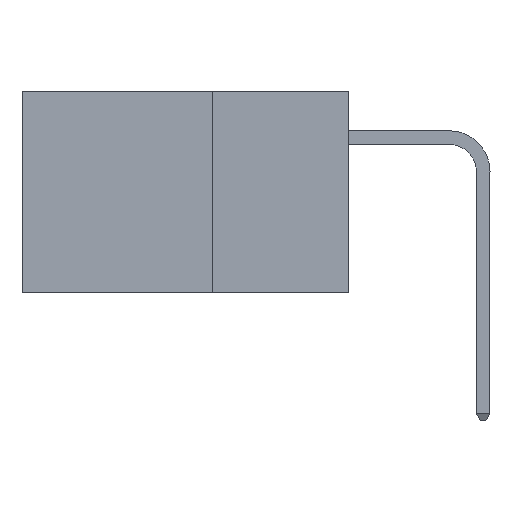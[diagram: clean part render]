
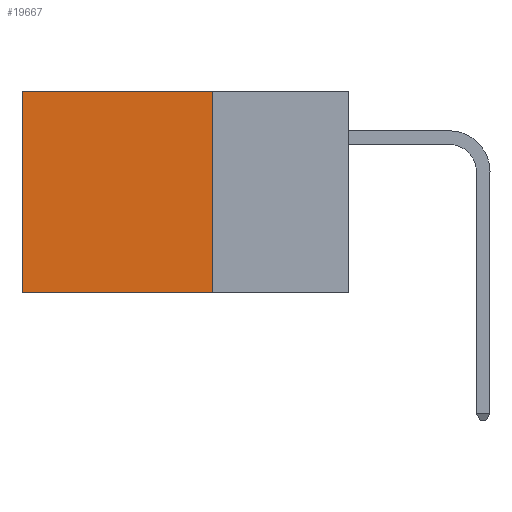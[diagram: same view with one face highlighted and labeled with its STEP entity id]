
A CAD part, left-side view. The second image highlights one B-rep face of the part: STEP entity #19667.
In plain terms, the highlighted planar face has unit normal (-1, 0, 0).
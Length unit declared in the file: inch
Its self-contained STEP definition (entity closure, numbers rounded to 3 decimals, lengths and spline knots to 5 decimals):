
#510 = VERTEX_POINT ( 'NONE', #16244 ) ;
#1344 = LINE ( 'NONE', #4701, #18742 ) ;
#1558 = CARTESIAN_POINT ( 'NONE',  ( 0.2875, 0.25, -0.37 ) ) ;
#2072 = CARTESIAN_POINT ( 'NONE',  ( 0.2875, 0.25, 0. ) ) ;
#2554 = ORIENTED_EDGE ( 'NONE', *, *, #17748, .T. ) ;
#4329 = LINE ( 'NONE', #9732, #13766 ) ;
#4585 = DIRECTION ( 'NONE',  ( 0., 1., 0. ) ) ;
#4683 = DIRECTION ( 'NONE',  ( 0., 0., -1. ) ) ;
#4701 = CARTESIAN_POINT ( 'NONE',  ( 0.2875, 0.25, -0.37 ) ) ;
#5340 = EDGE_CURVE ( 'NONE', #510, #19497, #20438, .T. ) ;
#6533 = CARTESIAN_POINT ( 'NONE',  ( 0.2875, 0.6, -0.37 ) ) ;
#7236 = DIRECTION ( 'NONE',  ( 0., 0., -1. ) ) ;
#8047 = DIRECTION ( 'NONE',  ( 0., 0., -1. ) ) ;
#8065 = FACE_OUTER_BOUND ( 'NONE', #16043, .T. ) ;
#8788 = VERTEX_POINT ( 'NONE', #9786 ) ;
#9732 = CARTESIAN_POINT ( 'NONE',  ( 0.2875, 0.6, 0. ) ) ;
#9786 = CARTESIAN_POINT ( 'NONE',  ( 0.2875, 0.6, 0. ) ) ;
#11157 = ORIENTED_EDGE ( 'NONE', *, *, #5340, .F. ) ;
#12168 = PLANE ( 'NONE',  #21202 ) ;
#13369 = ORIENTED_EDGE ( 'NONE', *, *, #16544, .T. ) ;
#13582 = VERTEX_POINT ( 'NONE', #6533 ) ;
#13766 = VECTOR ( 'NONE', #4683, 39.37008 ) ;
#14078 = VECTOR ( 'NONE', #4585, 39.37008 ) ;
#14238 = ORIENTED_EDGE ( 'NONE', *, *, #20639, .F. ) ;
#16010 = VECTOR ( 'NONE', #8047, 39.37008 ) ;
#16043 = EDGE_LOOP ( 'NONE', ( #2554, #14238, #11157, #13369 ) ) ;
#16244 = CARTESIAN_POINT ( 'NONE',  ( 0.2875, 0.25, 0. ) ) ;
#16259 = CARTESIAN_POINT ( 'NONE',  ( 0.2875, 0.25, 0. ) ) ;
#16544 = EDGE_CURVE ( 'NONE', #510, #8788, #18528, .T. ) ;
#17231 = DIRECTION ( 'NONE',  ( 1., 0., 0. ) ) ;
#17748 = EDGE_CURVE ( 'NONE', #8788, #13582, #4329, .T. ) ;
#18056 = CARTESIAN_POINT ( 'NONE',  ( 0.2875, 0.25, 0. ) ) ;
#18528 = LINE ( 'NONE', #16259, #14078 ) ;
#18742 = VECTOR ( 'NONE', #21382, 39.37008 ) ;
#19497 = VERTEX_POINT ( 'NONE', #1558 ) ;
#19667 = ADVANCED_FACE ( 'NONE', ( #8065 ), #12168, .F. ) ;
#20438 = LINE ( 'NONE', #18056, #16010 ) ;
#20639 = EDGE_CURVE ( 'NONE', #19497, #13582, #1344, .T. ) ;
#21202 = AXIS2_PLACEMENT_3D ( 'NONE', #2072, #17231, #7236 ) ;
#21382 = DIRECTION ( 'NONE',  ( 0., 1., 0. ) ) ;
